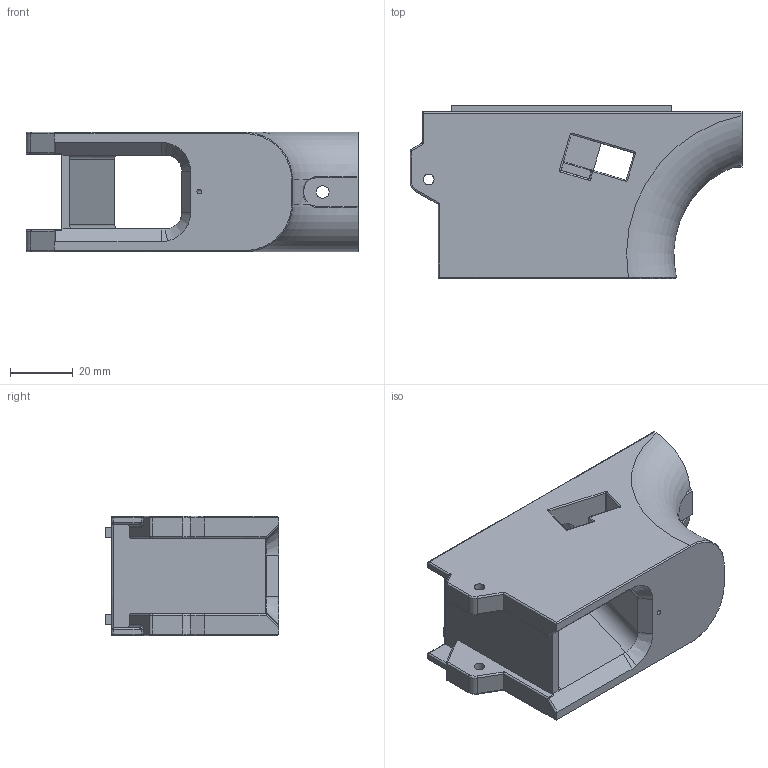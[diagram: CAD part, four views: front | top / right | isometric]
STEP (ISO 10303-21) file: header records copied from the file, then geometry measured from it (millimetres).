
FILE_DESCRIPTION (( 'STEP AP203' ), '1' );
FILE_NAME ('MOD9_magwell.STEP', '2020-06-10T05:00:04', ( '' ), ( '' ), 'SwSTEP 2.0', 'SolidWorks 2016', '' );
FILE_SCHEMA (( 'CONFIG_CONTROL_DESIGN' ));
Length unit declared in the file: millimetre
Products named in the file (1): MOD9_magwell
Bounding box: 105.51 x 55 x 38 mm (x, y, z)
Volume: 110345.2 mm3; surface area: 28185.9 mm2
Topology: 1 solids, 1 shells, 529 faces, 1430 edges, 909 vertices
Faces by surface type: bspline 264, plane 140, cylinder 98, torus 19, sphere 6, cone 2
Full cylindrical faces by diameter (mm): 1.5 x1, 3.4 x2, 4 x2
Entity records: 22963 total; most frequent: CARTESIAN_POINT 11447, ORIENTED_EDGE 2842, DIRECTION 1559, EDGE_CURVE 1421, VERTEX_POINT 909, VECTOR 719, LINE 719, EDGE_LOOP 560
